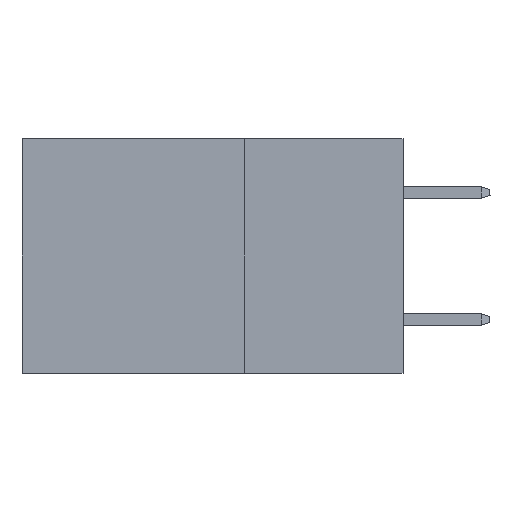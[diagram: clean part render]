
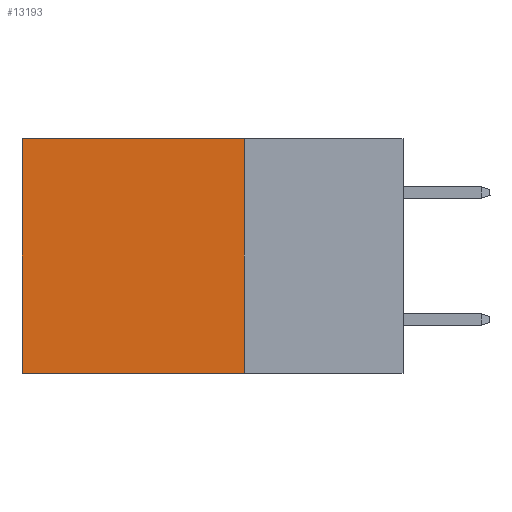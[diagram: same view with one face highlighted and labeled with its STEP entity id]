
A CAD part, left-side view. The second image highlights one B-rep face of the part: STEP entity #13193.
In plain terms, the highlighted planar face has unit normal (-1, 0, 0).
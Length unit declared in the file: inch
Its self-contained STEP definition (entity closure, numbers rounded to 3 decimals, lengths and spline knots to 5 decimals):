
#624 = AXIS2_PLACEMENT_3D ( 'NONE', #12526, #21410, #13080 ) ;
#785 = VECTOR ( 'NONE', #9484, 39.37008 ) ;
#1039 = DIRECTION ( 'NONE',  ( 0., 1., 0. ) ) ;
#1132 = VERTEX_POINT ( 'NONE', #5247 ) ;
#4164 = DIRECTION ( 'NONE',  ( 0., 1., 0. ) ) ;
#5016 = CARTESIAN_POINT ( 'NONE',  ( 0.2875, 0.25, 0. ) ) ;
#5214 = DIRECTION ( 'NONE',  ( 0., 0., -1. ) ) ;
#5247 = CARTESIAN_POINT ( 'NONE',  ( 0.2875, 0.6, 0. ) ) ;
#6722 = VECTOR ( 'NONE', #1039, 39.37008 ) ;
#6773 = LINE ( 'NONE', #35920, #785 ) ;
#9484 = DIRECTION ( 'NONE',  ( 0., 0., -1. ) ) ;
#10101 = CARTESIAN_POINT ( 'NONE',  ( 0.2875, 0.25, -0.37 ) ) ;
#10811 = LINE ( 'NONE', #5016, #37427 ) ;
#11538 = EDGE_CURVE ( 'NONE', #22034, #17473, #18412, .T. ) ;
#12117 = VERTEX_POINT ( 'NONE', #23354 ) ;
#12290 = EDGE_CURVE ( 'NONE', #12117, #1132, #36441, .T. ) ;
#12526 = CARTESIAN_POINT ( 'NONE',  ( 0.2875, 0.25, 0. ) ) ;
#13080 = DIRECTION ( 'NONE',  ( 0., 0., -1. ) ) ;
#13193 = ADVANCED_FACE ( 'NONE', ( #15424 ), #36274, .F. ) ;
#13500 = VECTOR ( 'NONE', #4164, 39.37008 ) ;
#15407 = ORIENTED_EDGE ( 'NONE', *, *, #11538, .F. ) ;
#15424 = FACE_OUTER_BOUND ( 'NONE', #30811, .T. ) ;
#17473 = VERTEX_POINT ( 'NONE', #23093 ) ;
#17857 = EDGE_CURVE ( 'NONE', #1132, #17473, #6773, .T. ) ;
#17904 = ORIENTED_EDGE ( 'NONE', *, *, #12290, .T. ) ;
#18412 = LINE ( 'NONE', #10101, #6722 ) ;
#21410 = DIRECTION ( 'NONE',  ( 1., 0., 0. ) ) ;
#22034 = VERTEX_POINT ( 'NONE', #26272 ) ;
#23093 = CARTESIAN_POINT ( 'NONE',  ( 0.2875, 0.6, -0.37 ) ) ;
#23354 = CARTESIAN_POINT ( 'NONE',  ( 0.2875, 0.25, 0. ) ) ;
#25477 = EDGE_CURVE ( 'NONE', #12117, #22034, #10811, .T. ) ;
#26272 = CARTESIAN_POINT ( 'NONE',  ( 0.2875, 0.25, -0.37 ) ) ;
#26458 = ORIENTED_EDGE ( 'NONE', *, *, #25477, .F. ) ;
#30412 = ORIENTED_EDGE ( 'NONE', *, *, #17857, .T. ) ;
#30621 = CARTESIAN_POINT ( 'NONE',  ( 0.2875, 0.25, 0. ) ) ;
#30811 = EDGE_LOOP ( 'NONE', ( #30412, #15407, #26458, #17904 ) ) ;
#35920 = CARTESIAN_POINT ( 'NONE',  ( 0.2875, 0.6, 0. ) ) ;
#36274 = PLANE ( 'NONE',  #624 ) ;
#36441 = LINE ( 'NONE', #30621, #13500 ) ;
#37427 = VECTOR ( 'NONE', #5214, 39.37008 ) ;
